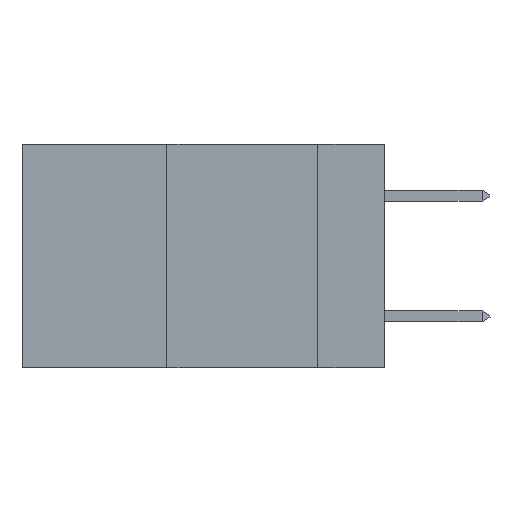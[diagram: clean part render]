
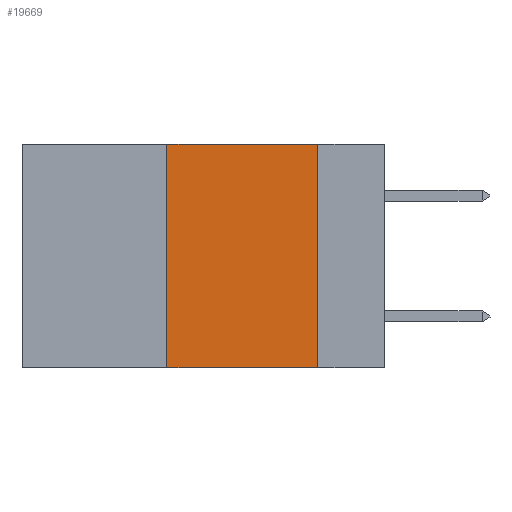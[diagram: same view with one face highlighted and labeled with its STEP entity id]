
A CAD part, left-side view. The second image highlights one B-rep face of the part: STEP entity #19669.
In plain terms, the highlighted planar face has unit normal (-1, 0, 0).
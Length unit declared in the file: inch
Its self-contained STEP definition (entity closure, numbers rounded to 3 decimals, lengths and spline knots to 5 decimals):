
#682 = VERTEX_POINT ( 'NONE', #2143 ) ;
#1640 = CARTESIAN_POINT ( 'NONE',  ( 0., 0.36, 0. ) ) ;
#1652 = ORIENTED_EDGE ( 'NONE', *, *, #7172, .F. ) ;
#2143 = CARTESIAN_POINT ( 'NONE',  ( 0., 0.36, -0.37 ) ) ;
#2715 = CARTESIAN_POINT ( 'NONE',  ( 0., 0.11, 0. ) ) ;
#2810 = DIRECTION ( 'NONE',  ( 0., 0., -1. ) ) ;
#3061 = FACE_OUTER_BOUND ( 'NONE', #12483, .T. ) ;
#3255 = VECTOR ( 'NONE', #6013, 39.37008 ) ;
#3393 = PLANE ( 'NONE',  #14900 ) ;
#4379 = ORIENTED_EDGE ( 'NONE', *, *, #4841, .F. ) ;
#4841 = EDGE_CURVE ( 'NONE', #682, #19005, #16870, .T. ) ;
#5133 = DIRECTION ( 'NONE',  ( 1., 0., 0. ) ) ;
#6013 = DIRECTION ( 'NONE',  ( 0., 0., 1. ) ) ;
#7172 = EDGE_CURVE ( 'NONE', #19005, #8788, #15747, .T. ) ;
#7905 = ORIENTED_EDGE ( 'NONE', *, *, #18756, .F. ) ;
#8541 = CARTESIAN_POINT ( 'NONE',  ( 0., 0.6, -0.37 ) ) ;
#8763 = LINE ( 'NONE', #13023, #21169 ) ;
#8788 = VERTEX_POINT ( 'NONE', #2715 ) ;
#10253 = DIRECTION ( 'NONE',  ( 0., -1., 0. ) ) ;
#11065 = LINE ( 'NONE', #8541, #16139 ) ;
#12336 = DIRECTION ( 'NONE',  ( 0., -1., 0. ) ) ;
#12483 = EDGE_LOOP ( 'NONE', ( #7905, #1652, #4379, #16869 ) ) ;
#13023 = CARTESIAN_POINT ( 'NONE',  ( 0., 0.11, 0. ) ) ;
#14060 = CARTESIAN_POINT ( 'NONE',  ( 0., 0.6, 0. ) ) ;
#14900 = AXIS2_PLACEMENT_3D ( 'NONE', #15348, #5133, #17038 ) ;
#15348 = CARTESIAN_POINT ( 'NONE',  ( 0., 0.6, 0. ) ) ;
#15747 = LINE ( 'NONE', #14060, #19116 ) ;
#16139 = VECTOR ( 'NONE', #10253, 39.37008 ) ;
#16869 = ORIENTED_EDGE ( 'NONE', *, *, #20186, .T. ) ;
#16870 = LINE ( 'NONE', #17852, #3255 ) ;
#16878 = CARTESIAN_POINT ( 'NONE',  ( 0., 0.11, -0.37 ) ) ;
#17038 = DIRECTION ( 'NONE',  ( 0., 0., -1. ) ) ;
#17852 = CARTESIAN_POINT ( 'NONE',  ( 0., 0.36, 0. ) ) ;
#18756 = EDGE_CURVE ( 'NONE', #8788, #19621, #8763, .T. ) ;
#19005 = VERTEX_POINT ( 'NONE', #1640 ) ;
#19116 = VECTOR ( 'NONE', #12336, 39.37008 ) ;
#19621 = VERTEX_POINT ( 'NONE', #16878 ) ;
#19669 = ADVANCED_FACE ( 'NONE', ( #3061 ), #3393, .F. ) ;
#20186 = EDGE_CURVE ( 'NONE', #682, #19621, #11065, .T. ) ;
#21169 = VECTOR ( 'NONE', #2810, 39.37008 ) ;
